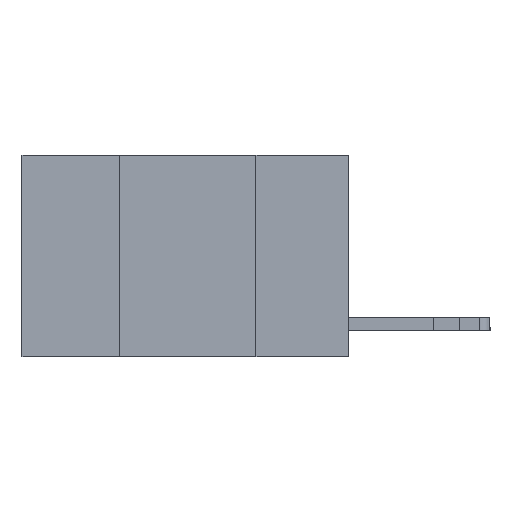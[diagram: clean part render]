
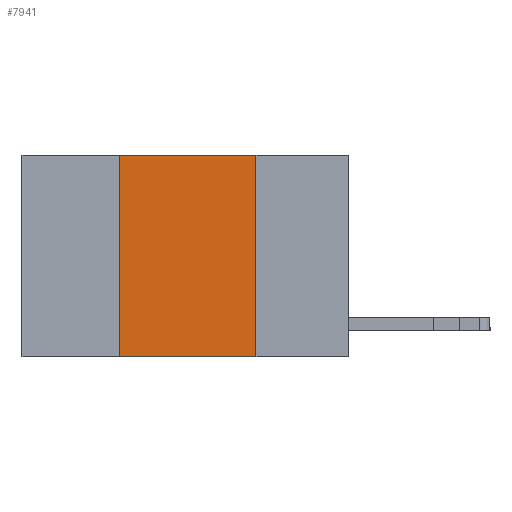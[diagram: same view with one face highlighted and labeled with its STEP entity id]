
A CAD part, left-side view. The second image highlights one B-rep face of the part: STEP entity #7941.
In plain terms, the highlighted planar face has unit normal (-1, 0, 0).
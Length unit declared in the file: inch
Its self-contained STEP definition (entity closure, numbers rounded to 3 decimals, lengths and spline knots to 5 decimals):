
#243 = EDGE_CURVE ( 'NONE', #2817, #2425, #2496, .T. ) ;
#1475 = DIRECTION ( 'NONE',  ( 0., -1., 0. ) ) ;
#1778 = CARTESIAN_POINT ( 'NONE',  ( 0., 0.42, -0.37 ) ) ;
#1804 = DIRECTION ( 'NONE',  ( 0., 0., 1. ) ) ;
#2196 = PLANE ( 'NONE',  #12557 ) ;
#2425 = VERTEX_POINT ( 'NONE', #2466 ) ;
#2466 = CARTESIAN_POINT ( 'NONE',  ( 0., 0.17, -0.37 ) ) ;
#2496 = LINE ( 'NONE', #11234, #7419 ) ;
#2817 = VERTEX_POINT ( 'NONE', #1778 ) ;
#3195 = VECTOR ( 'NONE', #6549, 39.37008 ) ;
#3868 = EDGE_CURVE ( 'NONE', #7634, #2425, #5056, .T. ) ;
#4327 = FACE_OUTER_BOUND ( 'NONE', #7651, .T. ) ;
#4387 = EDGE_CURVE ( 'NONE', #9188, #7634, #6609, .T. ) ;
#5056 = LINE ( 'NONE', #9001, #8397 ) ;
#5175 = DIRECTION ( 'NONE',  ( 0., 0., -1. ) ) ;
#5307 = CARTESIAN_POINT ( 'NONE',  ( 0., 0.42, 0. ) ) ;
#6359 = ORIENTED_EDGE ( 'NONE', *, *, #7614, .F. ) ;
#6534 = ORIENTED_EDGE ( 'NONE', *, *, #243, .T. ) ;
#6549 = DIRECTION ( 'NONE',  ( 0., -1., 0. ) ) ;
#6609 = LINE ( 'NONE', #7341, #3195 ) ;
#7341 = CARTESIAN_POINT ( 'NONE',  ( 0., 0.6, 0. ) ) ;
#7419 = VECTOR ( 'NONE', #1475, 39.37008 ) ;
#7614 = EDGE_CURVE ( 'NONE', #2817, #9188, #10407, .T. ) ;
#7634 = VERTEX_POINT ( 'NONE', #10660 ) ;
#7651 = EDGE_LOOP ( 'NONE', ( #7668, #8682, #6359, #6534 ) ) ;
#7668 = ORIENTED_EDGE ( 'NONE', *, *, #3868, .F. ) ;
#7941 = ADVANCED_FACE ( 'NONE', ( #4327 ), #2196, .F. ) ;
#8397 = VECTOR ( 'NONE', #10563, 39.37008 ) ;
#8682 = ORIENTED_EDGE ( 'NONE', *, *, #4387, .F. ) ;
#9001 = CARTESIAN_POINT ( 'NONE',  ( 0., 0.17, 0. ) ) ;
#9188 = VERTEX_POINT ( 'NONE', #5307 ) ;
#10407 = LINE ( 'NONE', #11622, #11164 ) ;
#10563 = DIRECTION ( 'NONE',  ( 0., 0., -1. ) ) ;
#10660 = CARTESIAN_POINT ( 'NONE',  ( 0., 0.17, 0. ) ) ;
#11164 = VECTOR ( 'NONE', #1804, 39.37008 ) ;
#11173 = DIRECTION ( 'NONE',  ( 1., 0., 0. ) ) ;
#11234 = CARTESIAN_POINT ( 'NONE',  ( 0., 0.6, -0.37 ) ) ;
#11622 = CARTESIAN_POINT ( 'NONE',  ( 0., 0.42, 0. ) ) ;
#12194 = CARTESIAN_POINT ( 'NONE',  ( 0., 0.6, 0. ) ) ;
#12557 = AXIS2_PLACEMENT_3D ( 'NONE', #12194, #11173, #5175 ) ;
